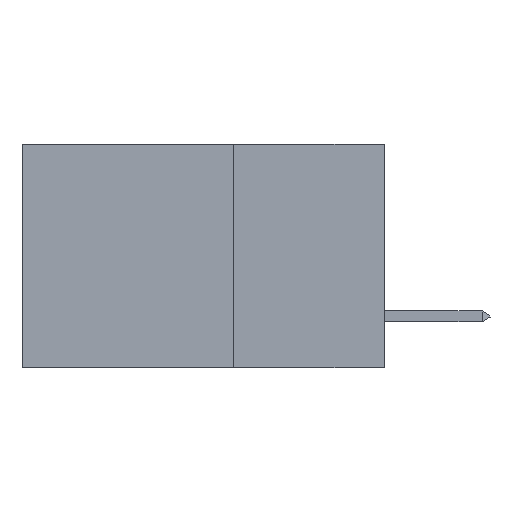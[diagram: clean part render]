
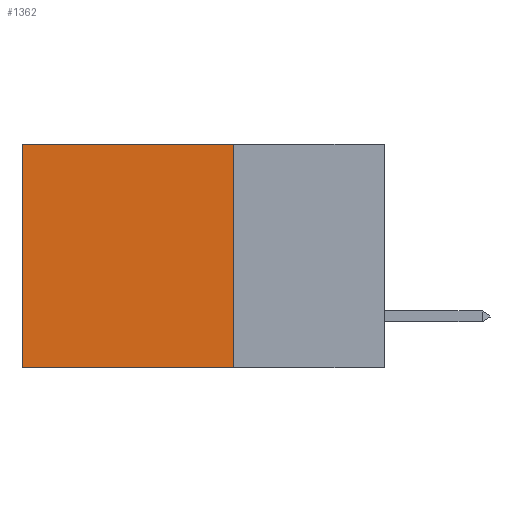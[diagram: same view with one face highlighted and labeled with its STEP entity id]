
A CAD part, left-side view. The second image highlights one B-rep face of the part: STEP entity #1362.
In plain terms, the highlighted planar face has unit normal (-1, 0, 0).
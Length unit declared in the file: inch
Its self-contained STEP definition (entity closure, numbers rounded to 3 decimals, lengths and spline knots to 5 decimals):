
#696 = VECTOR ( 'NONE', #15488, 39.37008 ) ;
#1362 = ADVANCED_FACE ( 'NONE', ( #8165 ), #2466, .F. ) ;
#1648 = CARTESIAN_POINT ( 'NONE',  ( 0.2875, 0.25, -0.37 ) ) ;
#1957 = VECTOR ( 'NONE', #1974, 39.37008 ) ;
#1974 = DIRECTION ( 'NONE',  ( 0., 1., 0. ) ) ;
#2466 = PLANE ( 'NONE',  #16780 ) ;
#3272 = CARTESIAN_POINT ( 'NONE',  ( 0.2875, 0.25, 0. ) ) ;
#3899 = CARTESIAN_POINT ( 'NONE',  ( 0.2875, 0.25, 0. ) ) ;
#4068 = LINE ( 'NONE', #3272, #696 ) ;
#4364 = CARTESIAN_POINT ( 'NONE',  ( 0.2875, 0.25, 0. ) ) ;
#4429 = EDGE_CURVE ( 'NONE', #16695, #10720, #7407, .T. ) ;
#4655 = ORIENTED_EDGE ( 'NONE', *, *, #12422, .F. ) ;
#5551 = DIRECTION ( 'NONE',  ( 0., 1., 0. ) ) ;
#6102 = EDGE_CURVE ( 'NONE', #10065, #16695, #8007, .T. ) ;
#7407 = LINE ( 'NONE', #11168, #10802 ) ;
#7881 = VERTEX_POINT ( 'NONE', #1648 ) ;
#8007 = LINE ( 'NONE', #8240, #12383 ) ;
#8165 = FACE_OUTER_BOUND ( 'NONE', #15737, .T. ) ;
#8240 = CARTESIAN_POINT ( 'NONE',  ( 0.2875, 0.25, 0. ) ) ;
#8640 = DIRECTION ( 'NONE',  ( 0., 0., -1. ) ) ;
#8872 = ORIENTED_EDGE ( 'NONE', *, *, #6102, .T. ) ;
#9274 = CARTESIAN_POINT ( 'NONE',  ( 0.2875, 0.6, 0. ) ) ;
#9362 = DIRECTION ( 'NONE',  ( 1., 0., 0. ) ) ;
#10065 = VERTEX_POINT ( 'NONE', #4364 ) ;
#10720 = VERTEX_POINT ( 'NONE', #12044 ) ;
#10802 = VECTOR ( 'NONE', #8640, 39.37008 ) ;
#11168 = CARTESIAN_POINT ( 'NONE',  ( 0.2875, 0.6, 0. ) ) ;
#11315 = ORIENTED_EDGE ( 'NONE', *, *, #16079, .F. ) ;
#11532 = ORIENTED_EDGE ( 'NONE', *, *, #4429, .T. ) ;
#12044 = CARTESIAN_POINT ( 'NONE',  ( 0.2875, 0.6, -0.37 ) ) ;
#12383 = VECTOR ( 'NONE', #5551, 39.37008 ) ;
#12422 = EDGE_CURVE ( 'NONE', #10065, #7881, #4068, .T. ) ;
#12575 = CARTESIAN_POINT ( 'NONE',  ( 0.2875, 0.25, -0.37 ) ) ;
#15488 = DIRECTION ( 'NONE',  ( 0., 0., -1. ) ) ;
#15737 = EDGE_LOOP ( 'NONE', ( #11532, #11315, #4655, #8872 ) ) ;
#16079 = EDGE_CURVE ( 'NONE', #7881, #10720, #16777, .T. ) ;
#16695 = VERTEX_POINT ( 'NONE', #9274 ) ;
#16777 = LINE ( 'NONE', #12575, #1957 ) ;
#16780 = AXIS2_PLACEMENT_3D ( 'NONE', #3899, #9362, #17104 ) ;
#17104 = DIRECTION ( 'NONE',  ( 0., 0., -1. ) ) ;
